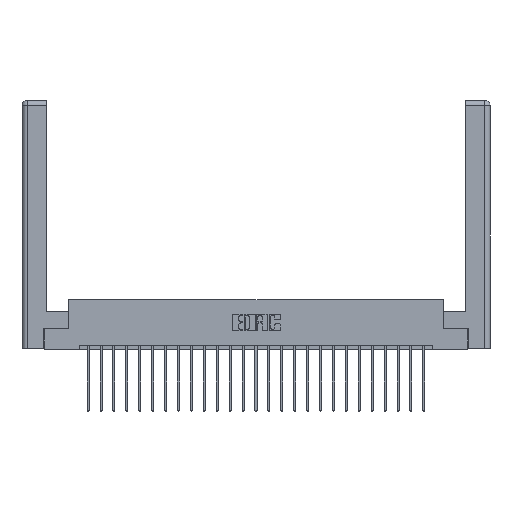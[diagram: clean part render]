
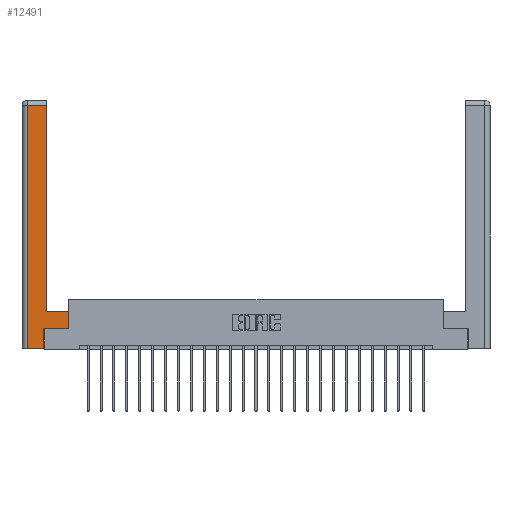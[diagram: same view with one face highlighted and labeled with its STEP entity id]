
A CAD part, top view. The second image highlights one B-rep face of the part: STEP entity #12491.
In plain terms, the highlighted planar face has unit normal (0, 0, 1).
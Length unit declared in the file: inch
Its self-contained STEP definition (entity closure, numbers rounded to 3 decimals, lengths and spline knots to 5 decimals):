
#172 = VECTOR ( 'NONE', #12701, 39.37008 ) ;
#405 = LINE ( 'NONE', #24703, #5679 ) ;
#436 = LINE ( 'NONE', #18731, #16481 ) ;
#1104 = ORIENTED_EDGE ( 'NONE', *, *, #14487, .T. ) ;
#1263 = CARTESIAN_POINT ( 'NONE',  ( 0.0615, 0., 0. ) ) ;
#1481 = DIRECTION ( 'NONE',  ( 1., 0., 0. ) ) ;
#1643 = EDGE_CURVE ( 'NONE', #14408, #15390, #10756, .T. ) ;
#1689 = ORIENTED_EDGE ( 'NONE', *, *, #8481, .T. ) ;
#1891 = DIRECTION ( 'NONE',  ( 0., 1., 0. ) ) ;
#1971 = AXIS2_PLACEMENT_3D ( 'NONE', #20041, #19884, #23984 ) ;
#3016 = VECTOR ( 'NONE', #15610, 39.37008 ) ;
#3319 = VECTOR ( 'NONE', #17117, 39.37008 ) ;
#3445 = FACE_OUTER_BOUND ( 'NONE', #9658, .T. ) ;
#3589 = LINE ( 'NONE', #18547, #172 ) ;
#3745 = CARTESIAN_POINT ( 'NONE',  ( 0.295, 3., 0. ) ) ;
#3756 = CARTESIAN_POINT ( 'NONE',  ( 0.265, 0., 0. ) ) ;
#4406 = VERTEX_POINT ( 'NONE', #10510 ) ;
#4485 = CARTESIAN_POINT ( 'NONE',  ( 0.565, 0.45, 0. ) ) ;
#4912 = CARTESIAN_POINT ( 'NONE',  ( 0.565, 0.245, 0. ) ) ;
#4998 = ORIENTED_EDGE ( 'NONE', *, *, #8037, .T. ) ;
#5009 = CARTESIAN_POINT ( 'NONE',  ( 0.565, 0.45, 0. ) ) ;
#5023 = DIRECTION ( 'NONE',  ( -1., 0., 0. ) ) ;
#5403 = ORIENTED_EDGE ( 'NONE', *, *, #9044, .T. ) ;
#5486 = EDGE_CURVE ( 'NONE', #15427, #15424, #21241, .T. ) ;
#5679 = VECTOR ( 'NONE', #7215, 39.37008 ) ;
#6107 = VERTEX_POINT ( 'NONE', #4485 ) ;
#7215 = DIRECTION ( 'NONE',  ( -1., 0., 0. ) ) ;
#7502 = CARTESIAN_POINT ( 'NONE',  ( 0.565, 0.245, 0. ) ) ;
#8037 = EDGE_CURVE ( 'NONE', #9624, #15427, #3589, .T. ) ;
#8481 = EDGE_CURVE ( 'NONE', #6107, #4406, #436, .T. ) ;
#8576 = LINE ( 'NONE', #5009, #3319 ) ;
#9044 = EDGE_CURVE ( 'NONE', #15390, #9624, #15538, .T. ) ;
#9068 = VECTOR ( 'NONE', #1891, 39.37008 ) ;
#9530 = VERTEX_POINT ( 'NONE', #19871 ) ;
#9624 = VERTEX_POINT ( 'NONE', #3756 ) ;
#9658 = EDGE_LOOP ( 'NONE', ( #24634, #11994, #13267, #5403, #4998, #18518, #1104, #1689 ) ) ;
#10510 = CARTESIAN_POINT ( 'NONE',  ( 0.295, 0.45, 0. ) ) ;
#10756 = LINE ( 'NONE', #11318, #3016 ) ;
#10784 = DIRECTION ( 'NONE',  ( 1., 0., 0. ) ) ;
#11069 = CARTESIAN_POINT ( 'NONE',  ( 0.265, 0., 0. ) ) ;
#11318 = CARTESIAN_POINT ( 'NONE',  ( 0.0615, 0., 0. ) ) ;
#11994 = ORIENTED_EDGE ( 'NONE', *, *, #25089, .T. ) ;
#12457 = VECTOR ( 'NONE', #1481, 39.37008 ) ;
#12491 = ADVANCED_FACE ( 'NONE', ( #3445 ), #16130, .F. ) ;
#12701 = DIRECTION ( 'NONE',  ( 0., 1., 0. ) ) ;
#13223 = VECTOR ( 'NONE', #10784, 39.37008 ) ;
#13267 = ORIENTED_EDGE ( 'NONE', *, *, #1643, .T. ) ;
#14408 = VERTEX_POINT ( 'NONE', #18193 ) ;
#14487 = EDGE_CURVE ( 'NONE', #15424, #6107, #8576, .T. ) ;
#15390 = VERTEX_POINT ( 'NONE', #1263 ) ;
#15424 = VERTEX_POINT ( 'NONE', #7502 ) ;
#15427 = VERTEX_POINT ( 'NONE', #19047 ) ;
#15538 = LINE ( 'NONE', #11069, #12457 ) ;
#15610 = DIRECTION ( 'NONE',  ( 0., -1., 0. ) ) ;
#16130 = PLANE ( 'NONE',  #1971 ) ;
#16481 = VECTOR ( 'NONE', #5023, 39.37008 ) ;
#16759 = LINE ( 'NONE', #3745, #9068 ) ;
#17074 = EDGE_CURVE ( 'NONE', #4406, #9530, #16759, .T. ) ;
#17117 = DIRECTION ( 'NONE',  ( 0., 1., 0. ) ) ;
#18193 = CARTESIAN_POINT ( 'NONE',  ( 0.0615, 2.94, 0. ) ) ;
#18518 = ORIENTED_EDGE ( 'NONE', *, *, #5486, .T. ) ;
#18547 = CARTESIAN_POINT ( 'NONE',  ( 0.265, 0.245, 0. ) ) ;
#18731 = CARTESIAN_POINT ( 'NONE',  ( 0.295, 0.45, 0. ) ) ;
#19047 = CARTESIAN_POINT ( 'NONE',  ( 0.265, 0.245, 0. ) ) ;
#19871 = CARTESIAN_POINT ( 'NONE',  ( 0.295, 2.94, 0. ) ) ;
#19884 = DIRECTION ( 'NONE',  ( 0., 0., -1. ) ) ;
#20041 = CARTESIAN_POINT ( 'NONE',  ( 0., 0., 0. ) ) ;
#21241 = LINE ( 'NONE', #4912, #13223 ) ;
#23984 = DIRECTION ( 'NONE',  ( -1., 0., 0. ) ) ;
#24634 = ORIENTED_EDGE ( 'NONE', *, *, #17074, .T. ) ;
#24703 = CARTESIAN_POINT ( 'NONE',  ( 0.0615, 2.94, 0. ) ) ;
#25089 = EDGE_CURVE ( 'NONE', #9530, #14408, #405, .T. ) ;
